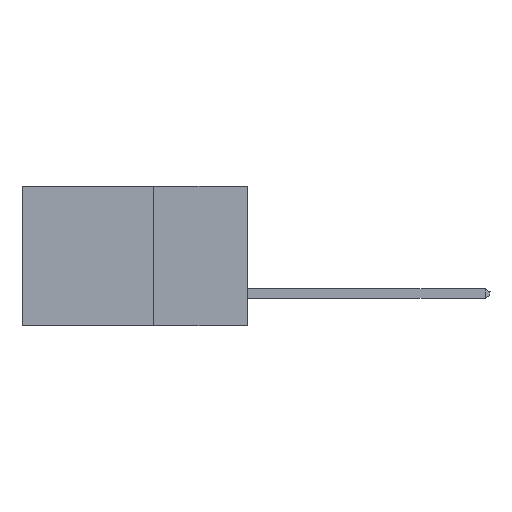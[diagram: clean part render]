
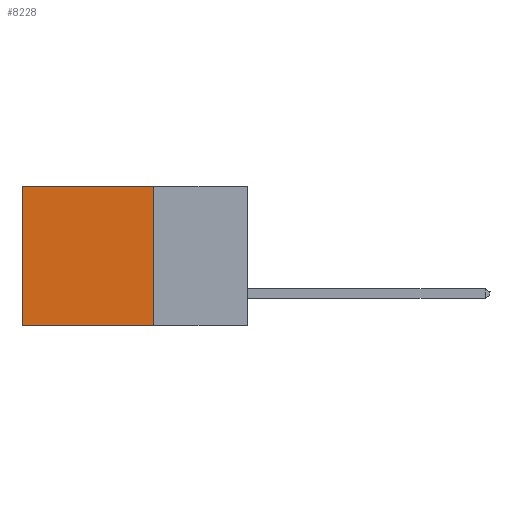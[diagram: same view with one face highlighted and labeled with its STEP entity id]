
A CAD part, left-side view. The second image highlights one B-rep face of the part: STEP entity #8228.
In plain terms, the highlighted planar face has unit normal (-1, 0, 0).
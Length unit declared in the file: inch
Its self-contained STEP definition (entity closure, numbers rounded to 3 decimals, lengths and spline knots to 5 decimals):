
#2222 = EDGE_CURVE ( 'NONE', #2306, #2992, #5812, .T. ) ;
#2306 = VERTEX_POINT ( 'NONE', #13411 ) ;
#2408 = DIRECTION ( 'NONE',  ( 0., 1., 0. ) ) ;
#2958 = DIRECTION ( 'NONE',  ( 1., 0., 0. ) ) ;
#2992 = VERTEX_POINT ( 'NONE', #4002 ) ;
#3575 = CARTESIAN_POINT ( 'NONE',  ( 0.2615, 0.25, -0.37 ) ) ;
#4002 = CARTESIAN_POINT ( 'NONE',  ( 0.2615, 0.25, -0.37 ) ) ;
#4215 = PLANE ( 'NONE',  #11069 ) ;
#4291 = CARTESIAN_POINT ( 'NONE',  ( 0.2615, 0.25, -0.37 ) ) ;
#4769 = ORIENTED_EDGE ( 'NONE', *, *, #6585, .F. ) ;
#5029 = EDGE_CURVE ( 'NONE', #10591, #12127, #13486, .T. ) ;
#5075 = EDGE_CURVE ( 'NONE', #2306, #10591, #6877, .T. ) ;
#5363 = FACE_OUTER_BOUND ( 'NONE', #7114, .T. ) ;
#5515 = DIRECTION ( 'NONE',  ( 0., 0., -1. ) ) ;
#5812 = LINE ( 'NONE', #11248, #8425 ) ;
#6266 = VECTOR ( 'NONE', #12934, 39.37008 ) ;
#6585 = EDGE_CURVE ( 'NONE', #2992, #12127, #14194, .T. ) ;
#6877 = LINE ( 'NONE', #12692, #6266 ) ;
#7054 = VECTOR ( 'NONE', #2408, 39.37008 ) ;
#7114 = EDGE_LOOP ( 'NONE', ( #8233, #4769, #13935, #15249 ) ) ;
#8228 = ADVANCED_FACE ( 'NONE', ( #5363 ), #4215, .F. ) ;
#8233 = ORIENTED_EDGE ( 'NONE', *, *, #5029, .T. ) ;
#8425 = VECTOR ( 'NONE', #11017, 39.37008 ) ;
#8760 = VECTOR ( 'NONE', #8829, 39.37008 ) ;
#8761 = CARTESIAN_POINT ( 'NONE',  ( 0.2615, 0.6, -0.37 ) ) ;
#8829 = DIRECTION ( 'NONE',  ( 0., 0., -1. ) ) ;
#10591 = VERTEX_POINT ( 'NONE', #13015 ) ;
#11017 = DIRECTION ( 'NONE',  ( 0., 0., -1. ) ) ;
#11069 = AXIS2_PLACEMENT_3D ( 'NONE', #4291, #2958, #5515 ) ;
#11248 = CARTESIAN_POINT ( 'NONE',  ( 0.2615, 0.25, -0.37 ) ) ;
#12127 = VERTEX_POINT ( 'NONE', #8761 ) ;
#12692 = CARTESIAN_POINT ( 'NONE',  ( 0.2615, 0.25, 0. ) ) ;
#12934 = DIRECTION ( 'NONE',  ( 0., 1., 0. ) ) ;
#13015 = CARTESIAN_POINT ( 'NONE',  ( 0.2615, 0.6, 0. ) ) ;
#13411 = CARTESIAN_POINT ( 'NONE',  ( 0.2615, 0.25, 0. ) ) ;
#13486 = LINE ( 'NONE', #14719, #8760 ) ;
#13935 = ORIENTED_EDGE ( 'NONE', *, *, #2222, .F. ) ;
#14194 = LINE ( 'NONE', #3575, #7054 ) ;
#14719 = CARTESIAN_POINT ( 'NONE',  ( 0.2615, 0.6, -0.37 ) ) ;
#15249 = ORIENTED_EDGE ( 'NONE', *, *, #5075, .T. ) ;
